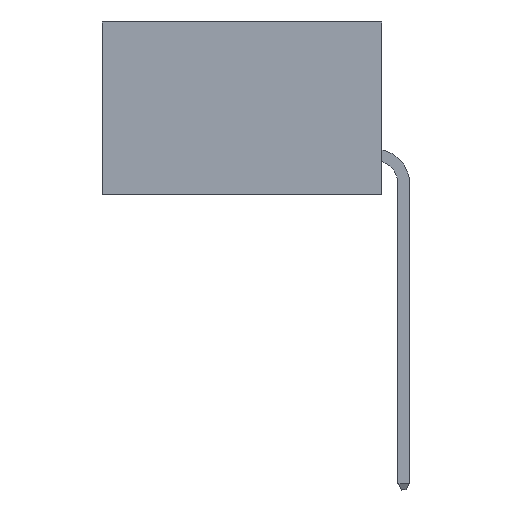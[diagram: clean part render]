
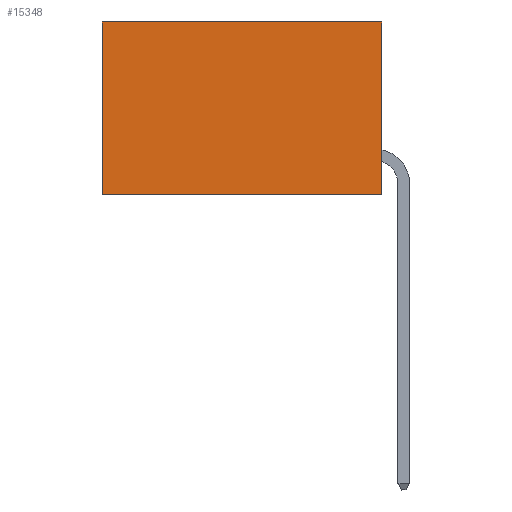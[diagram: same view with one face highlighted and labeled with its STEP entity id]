
A CAD part, left-side view. The second image highlights one B-rep face of the part: STEP entity #15348.
In plain terms, the highlighted planar face has unit normal (-1, 0, 0).
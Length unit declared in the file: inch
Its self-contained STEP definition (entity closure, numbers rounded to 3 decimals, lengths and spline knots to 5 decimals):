
#573 = CARTESIAN_POINT ( 'NONE',  ( 0.2875, 0.6, 0. ) ) ;
#1207 = VECTOR ( 'NONE', #19573, 39.37008 ) ;
#2199 = CARTESIAN_POINT ( 'NONE',  ( 0.2875, 0., -0.37 ) ) ;
#2384 = CARTESIAN_POINT ( 'NONE',  ( 0.2875, 0.6, -0.37 ) ) ;
#3709 = VERTEX_POINT ( 'NONE', #5488 ) ;
#3983 = ORIENTED_EDGE ( 'NONE', *, *, #32492, .T. ) ;
#4481 = CARTESIAN_POINT ( 'NONE',  ( 0.2875, 0., 0. ) ) ;
#5203 = ORIENTED_EDGE ( 'NONE', *, *, #6053, .T. ) ;
#5488 = CARTESIAN_POINT ( 'NONE',  ( 0.2875, 0.6, 0. ) ) ;
#5490 = CARTESIAN_POINT ( 'NONE',  ( 0.2875, 0., 0. ) ) ;
#6053 = EDGE_CURVE ( 'NONE', #22995, #3709, #15512, .T. ) ;
#8299 = VERTEX_POINT ( 'NONE', #31409 ) ;
#8644 = ORIENTED_EDGE ( 'NONE', *, *, #15219, .F. ) ;
#9236 = EDGE_LOOP ( 'NONE', ( #3983, #8644, #16692, #5203 ) ) ;
#10190 = LINE ( 'NONE', #573, #1207 ) ;
#11409 = AXIS2_PLACEMENT_3D ( 'NONE', #20249, #18341, #34351 ) ;
#11585 = VECTOR ( 'NONE', #16293, 39.37008 ) ;
#14795 = PLANE ( 'NONE',  #11409 ) ;
#15219 = EDGE_CURVE ( 'NONE', #8299, #26789, #18994, .T. ) ;
#15348 = ADVANCED_FACE ( 'NONE', ( #19813 ), #14795, .F. ) ;
#15512 = LINE ( 'NONE', #30524, #24381 ) ;
#15621 = VECTOR ( 'NONE', #18809, 39.37008 ) ;
#16293 = DIRECTION ( 'NONE',  ( 0., 0., -1. ) ) ;
#16692 = ORIENTED_EDGE ( 'NONE', *, *, #28009, .F. ) ;
#17249 = DIRECTION ( 'NONE',  ( 0., 1., 0. ) ) ;
#18341 = DIRECTION ( 'NONE',  ( 1., 0., 0. ) ) ;
#18740 = LINE ( 'NONE', #5490, #11585 ) ;
#18809 = DIRECTION ( 'NONE',  ( 0., 1., 0. ) ) ;
#18994 = LINE ( 'NONE', #2199, #15621 ) ;
#19573 = DIRECTION ( 'NONE',  ( 0., 0., -1. ) ) ;
#19813 = FACE_OUTER_BOUND ( 'NONE', #9236, .T. ) ;
#20249 = CARTESIAN_POINT ( 'NONE',  ( 0.2875, 0., 0. ) ) ;
#22995 = VERTEX_POINT ( 'NONE', #4481 ) ;
#24381 = VECTOR ( 'NONE', #17249, 39.37008 ) ;
#26789 = VERTEX_POINT ( 'NONE', #2384 ) ;
#28009 = EDGE_CURVE ( 'NONE', #22995, #8299, #18740, .T. ) ;
#30524 = CARTESIAN_POINT ( 'NONE',  ( 0.2875, 0., 0. ) ) ;
#31409 = CARTESIAN_POINT ( 'NONE',  ( 0.2875, 0., -0.37 ) ) ;
#32492 = EDGE_CURVE ( 'NONE', #3709, #26789, #10190, .T. ) ;
#34351 = DIRECTION ( 'NONE',  ( 0., 0., -1. ) ) ;
